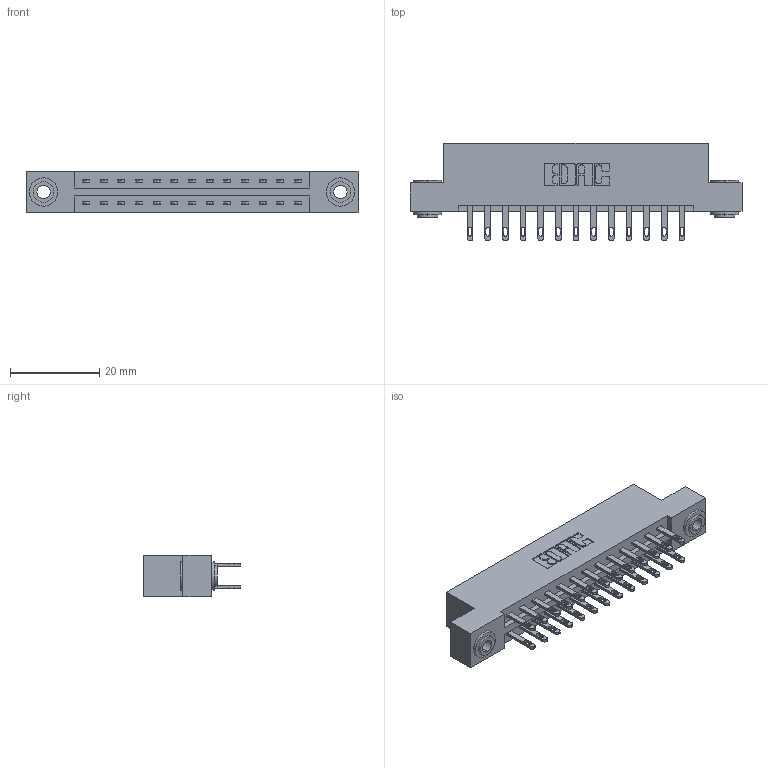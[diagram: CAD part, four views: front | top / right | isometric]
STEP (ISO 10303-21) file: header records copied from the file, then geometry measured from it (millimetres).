
FILE_DESCRIPTION (( 'STEP AP203' ), '1' );
FILE_NAME ('887-026-500-203.STEP', '2020-09-20T19:33:58', ( '' ), ( '' ), 'SwSTEP 2.0', 'SolidWorks 2020', '' );
FILE_SCHEMA (( 'CONFIG_CONTROL_DESIGN' ));
Length unit declared in the file: inch
Products named in the file (4): 837 Part_Flush Mounting Lugs - 0.156 Dia-TH; 345-250-002_345-250-002-102; 345-292-001_345-293-100; 887-026-500-203
Assembly tree (29 placements, depth 2):
  887-026-500-203
    837 Part_Flush Mounting Lugs - 0.156 Dia-TH
    345-292-001_345-293-100  x26
    345-250-002_345-250-002-102  x2
Bounding box: 74.52 x 21.85 x 9.4 mm (x, y, z)
Volume: 7566.7 mm3; surface area: 8785.4 mm2
Topology: 29 solids, 29 shells, 1452 faces, 4365 edges, 2906 vertices
Faces by surface type: plane 912, cylinder 532, cone 8
Entity records: 14410 total; most frequent: CARTESIAN_POINT 2425, ORIENTED_EDGE 2354, DIRECTION 2151, EDGE_CURVE 1177, VECTOR 1021, LINE 1021, VERTEX_POINT 782, AXIS2_PLACEMENT_3D 565
